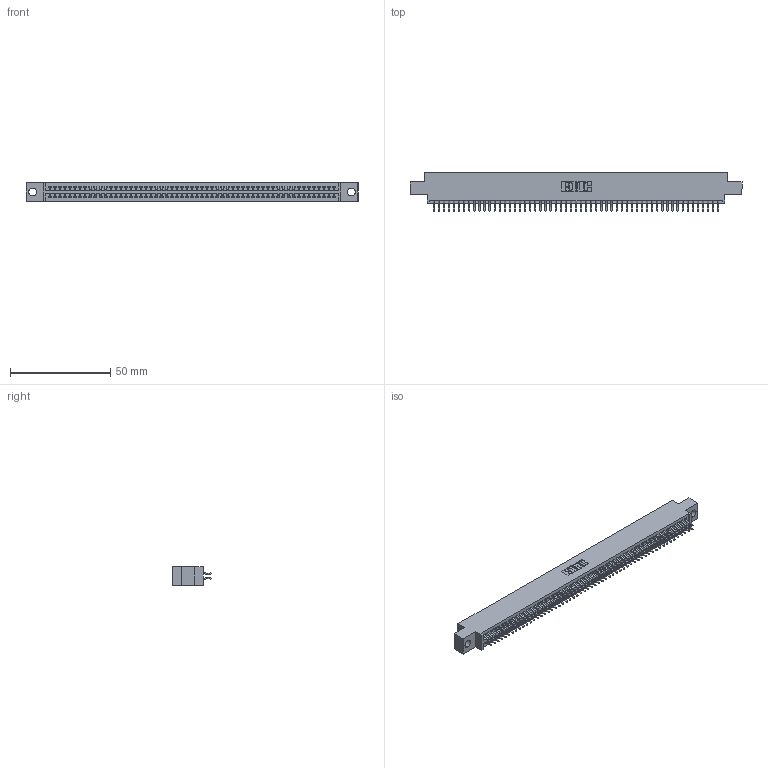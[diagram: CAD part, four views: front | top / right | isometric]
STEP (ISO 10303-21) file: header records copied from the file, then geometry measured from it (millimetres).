
FILE_DESCRIPTION (( 'STEP AP203' ), '1' );
FILE_NAME ('345-114-556-804.STEP', '2018-10-18T15:45:14', ( '' ), ( '' ), 'SwSTEP 2.0', 'SolidWorks 2016', '' );
FILE_SCHEMA (( 'CONFIG_CONTROL_DESIGN' ));
Length unit declared in the file: inch
Products named in the file (3): 345-292-001_556 Tail; 345 Part_0.170 Offset - 0.156 Dia-TH; 345-114-556-804
Assembly tree (115 placements, depth 2):
  345-114-556-804
    345 Part_0.170 Offset - 0.156 Dia-TH
    345-292-001_556 Tail  x114
Bounding box: 165.99 x 19.24 x 9.4 mm (x, y, z)
Volume: 16057.8 mm3; surface area: 23885.5 mm2
Topology: 115 solids, 115 shells, 6514 faces, 19391 edges, 12774 vertices
Faces by surface type: plane 4302, cylinder 2212
Entity records: 43059 total; most frequent: CARTESIAN_POINT 7220, ORIENTED_EDGE 7142, DIRECTION 6335, EDGE_CURVE 3571, VECTOR 3203, LINE 3203, VERTEX_POINT 2378, AXIS2_PLACEMENT_3D 1566
